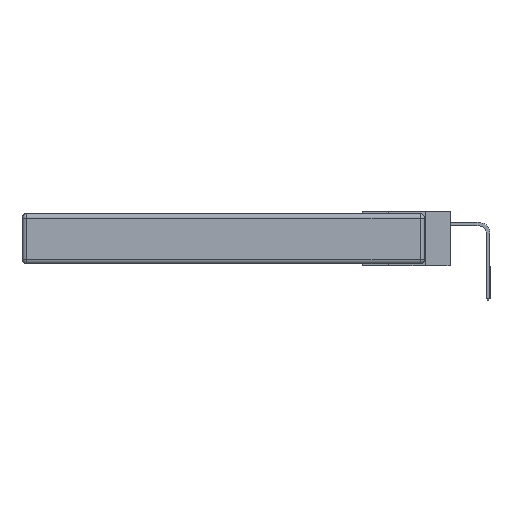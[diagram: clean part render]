
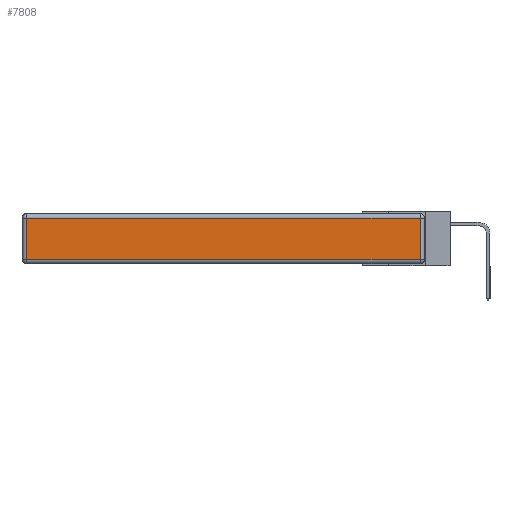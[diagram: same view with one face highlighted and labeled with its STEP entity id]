
A CAD part, left-side view. The second image highlights one B-rep face of the part: STEP entity #7808.
In plain terms, the highlighted planar face has unit normal (-1, 0, 0).
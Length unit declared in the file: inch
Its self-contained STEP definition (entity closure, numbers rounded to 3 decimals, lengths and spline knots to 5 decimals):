
#568 = CARTESIAN_POINT ( 'NONE',  ( 0., 2.75, -0.03 ) ) ;
#2157 = FACE_OUTER_BOUND ( 'NONE', #4332, .T. ) ;
#3067 = PLANE ( 'NONE',  #14701 ) ;
#3165 = EDGE_CURVE ( 'NONE', #7556, #19999, #30027, .T. ) ;
#4332 = EDGE_LOOP ( 'NONE', ( #21041, #8396, #29652, #24767 ) ) ;
#6183 = VECTOR ( 'NONE', #19012, 39.37008 ) ;
#6290 = CARTESIAN_POINT ( 'NONE',  ( 0., 2.72, -0.343 ) ) ;
#7274 = VECTOR ( 'NONE', #19296, 39.37008 ) ;
#7556 = VERTEX_POINT ( 'NONE', #11340 ) ;
#7808 = ADVANCED_FACE ( 'NONE', ( #2157 ), #3067, .T. ) ;
#8396 = ORIENTED_EDGE ( 'NONE', *, *, #12346, .T. ) ;
#9662 = CARTESIAN_POINT ( 'NONE',  ( 0., 0.03, -0.313 ) ) ;
#11340 = CARTESIAN_POINT ( 'NONE',  ( 0., 2.72, -0.313 ) ) ;
#12050 = CARTESIAN_POINT ( 'NONE',  ( 0., 0.03, -0.03 ) ) ;
#12346 = EDGE_CURVE ( 'NONE', #19999, #19946, #28623, .T. ) ;
#14312 = VERTEX_POINT ( 'NONE', #27893 ) ;
#14701 = AXIS2_PLACEMENT_3D ( 'NONE', #26391, #26616, #19490 ) ;
#16585 = CARTESIAN_POINT ( 'NONE',  ( 0., 0.03, -0.343 ) ) ;
#16832 = CARTESIAN_POINT ( 'NONE',  ( 0., 0., -0.313 ) ) ;
#17979 = DIRECTION ( 'NONE',  ( 0., 0., -1. ) ) ;
#19012 = DIRECTION ( 'NONE',  ( 0., 0., 1. ) ) ;
#19296 = DIRECTION ( 'NONE',  ( 0., 1., 0. ) ) ;
#19400 = LINE ( 'NONE', #6290, #29364 ) ;
#19490 = DIRECTION ( 'NONE',  ( 0., 0., 1. ) ) ;
#19582 = EDGE_CURVE ( 'NONE', #19946, #14312, #20483, .T. ) ;
#19946 = VERTEX_POINT ( 'NONE', #12050 ) ;
#19999 = VERTEX_POINT ( 'NONE', #9662 ) ;
#20483 = LINE ( 'NONE', #568, #7274 ) ;
#21041 = ORIENTED_EDGE ( 'NONE', *, *, #3165, .T. ) ;
#23730 = VECTOR ( 'NONE', #26510, 39.37008 ) ;
#23986 = EDGE_CURVE ( 'NONE', #14312, #7556, #19400, .T. ) ;
#24767 = ORIENTED_EDGE ( 'NONE', *, *, #23986, .T. ) ;
#26391 = CARTESIAN_POINT ( 'NONE',  ( 0., 0., -0.343 ) ) ;
#26510 = DIRECTION ( 'NONE',  ( 0., -1., 0. ) ) ;
#26616 = DIRECTION ( 'NONE',  ( -1., 0., 0. ) ) ;
#27893 = CARTESIAN_POINT ( 'NONE',  ( 0., 2.72, -0.03 ) ) ;
#28623 = LINE ( 'NONE', #16585, #6183 ) ;
#29364 = VECTOR ( 'NONE', #17979, 39.37008 ) ;
#29652 = ORIENTED_EDGE ( 'NONE', *, *, #19582, .T. ) ;
#30027 = LINE ( 'NONE', #16832, #23730 ) ;
